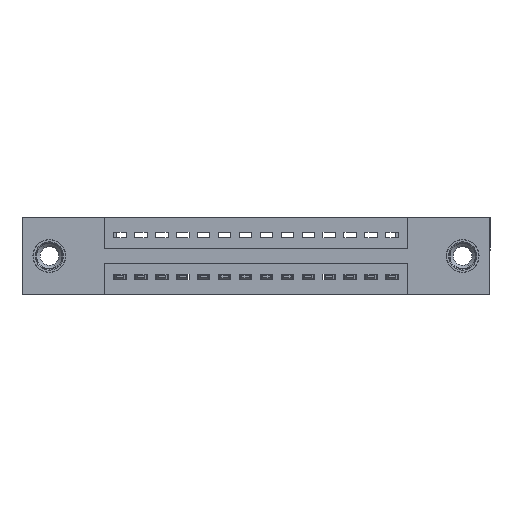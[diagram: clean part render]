
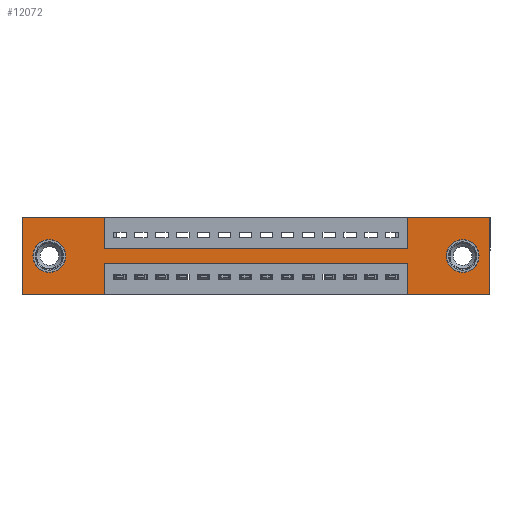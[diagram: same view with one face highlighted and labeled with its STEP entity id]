
A CAD part, front view. The second image highlights one B-rep face of the part: STEP entity #12072.
In plain terms, the highlighted planar face has unit normal (0, -1, 0).
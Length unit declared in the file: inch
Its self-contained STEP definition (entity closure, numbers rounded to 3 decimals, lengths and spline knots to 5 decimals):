
#70 = DIRECTION ( 'NONE',  ( 0., 1., 0. ) ) ;
#460 = AXIS2_PLACEMENT_3D ( 'NONE', #9441, #3684, #16946 ) ;
#713 = ORIENTED_EDGE ( 'NONE', *, *, #5972, .T. ) ;
#803 = ORIENTED_EDGE ( 'NONE', *, *, #4279, .F. ) ;
#848 = VERTEX_POINT ( 'NONE', #864 ) ;
#864 = CARTESIAN_POINT ( 'NONE',  ( 0., 0., 0. ) ) ;
#1004 = CARTESIAN_POINT ( 'NONE',  ( 0.3925, 0., -0.15 ) ) ;
#1243 = CARTESIAN_POINT ( 'NONE',  ( 2.235, 0., -0.37 ) ) ;
#1467 = ORIENTED_EDGE ( 'NONE', *, *, #2951, .F. ) ;
#1725 = VERTEX_POINT ( 'NONE', #14368 ) ;
#1738 = ORIENTED_EDGE ( 'NONE', *, *, #15918, .F. ) ;
#1948 = VERTEX_POINT ( 'NONE', #15063 ) ;
#2134 = CIRCLE ( 'NONE', #8075, 0.078 ) ;
#2428 = AXIS2_PLACEMENT_3D ( 'NONE', #12724, #17156, #8420 ) ;
#2469 = DIRECTION ( 'NONE',  ( 0., 0., 1. ) ) ;
#2610 = VECTOR ( 'NONE', #10086, 39.37008 ) ;
#2672 = CARTESIAN_POINT ( 'NONE',  ( 0.3925, 0., 0. ) ) ;
#2743 = VERTEX_POINT ( 'NONE', #13934 ) ;
#2900 = DIRECTION ( 'NONE',  ( 0., 0., 1. ) ) ;
#2901 = CARTESIAN_POINT ( 'NONE',  ( 1.8425, 0., -0.15 ) ) ;
#2913 = VECTOR ( 'NONE', #6463, 39.37008 ) ;
#2951 = EDGE_CURVE ( 'NONE', #15382, #3412, #18261, .T. ) ;
#3011 = CARTESIAN_POINT ( 'NONE',  ( 2.105, 0., -0.107 ) ) ;
#3070 = CARTESIAN_POINT ( 'NONE',  ( 1.8425, 0., -0.37 ) ) ;
#3412 = VERTEX_POINT ( 'NONE', #1243 ) ;
#3511 = DIRECTION ( 'NONE',  ( 0., 0., 1. ) ) ;
#3582 = EDGE_LOOP ( 'NONE', ( #16602, #17034 ) ) ;
#3594 = LINE ( 'NONE', #12085, #9097 ) ;
#3684 = DIRECTION ( 'NONE',  ( 0., -1., 0. ) ) ;
#3958 = DIRECTION ( 'NONE',  ( 0., 1., 0. ) ) ;
#4279 = EDGE_CURVE ( 'NONE', #848, #5965, #17296, .T. ) ;
#4366 = AXIS2_PLACEMENT_3D ( 'NONE', #18136, #3958, #3511 ) ;
#4417 = VECTOR ( 'NONE', #6159, 39.37008 ) ;
#4729 = VERTEX_POINT ( 'NONE', #15032 ) ;
#4902 = EDGE_CURVE ( 'NONE', #5724, #7267, #16792, .T. ) ;
#4928 = CARTESIAN_POINT ( 'NONE',  ( 0., 0., 0. ) ) ;
#5136 = VERTEX_POINT ( 'NONE', #2901 ) ;
#5249 = VERTEX_POINT ( 'NONE', #10340 ) ;
#5515 = CARTESIAN_POINT ( 'NONE',  ( 0.3925, 0., -0.22 ) ) ;
#5569 = DIRECTION ( 'NONE',  ( 0., 0., -1. ) ) ;
#5599 = VECTOR ( 'NONE', #14789, 39.37008 ) ;
#5714 = CARTESIAN_POINT ( 'NONE',  ( 0.3925, 0., 0. ) ) ;
#5724 = VERTEX_POINT ( 'NONE', #3070 ) ;
#5726 = CARTESIAN_POINT ( 'NONE',  ( 0.3925, 0., -0.15 ) ) ;
#5784 = FACE_BOUND ( 'NONE', #3582, .T. ) ;
#5814 = VECTOR ( 'NONE', #12591, 39.37008 ) ;
#5965 = VERTEX_POINT ( 'NONE', #2672 ) ;
#5972 = EDGE_CURVE ( 'NONE', #16766, #5249, #2134, .T. ) ;
#6159 = DIRECTION ( 'NONE',  ( -1., 0., 0. ) ) ;
#6307 = LINE ( 'NONE', #17658, #9524 ) ;
#6326 = CIRCLE ( 'NONE', #2428, 0.078 ) ;
#6414 = EDGE_CURVE ( 'NONE', #3412, #5724, #12609, .T. ) ;
#6463 = DIRECTION ( 'NONE',  ( -1., 0., 0. ) ) ;
#6726 = PLANE ( 'NONE',  #460 ) ;
#7267 = VERTEX_POINT ( 'NONE', #7624 ) ;
#7563 = VECTOR ( 'NONE', #2469, 39.37008 ) ;
#7624 = CARTESIAN_POINT ( 'NONE',  ( 1.8425, 0., -0.22 ) ) ;
#7673 = DIRECTION ( 'NONE',  ( -1., 0., 0. ) ) ;
#8075 = AXIS2_PLACEMENT_3D ( 'NONE', #12919, #17288, #15666 ) ;
#8339 = LINE ( 'NONE', #1004, #5814 ) ;
#8417 = VERTEX_POINT ( 'NONE', #14760 ) ;
#8420 = DIRECTION ( 'NONE',  ( 0., 0., -1. ) ) ;
#8852 = EDGE_LOOP ( 'NONE', ( #18480, #1738, #18056, #14288, #1467, #11668, #10074, #9271, #14047, #803, #10194, #9444 ) ) ;
#9030 = FACE_OUTER_BOUND ( 'NONE', #8852, .T. ) ;
#9097 = VECTOR ( 'NONE', #9306, 39.37008 ) ;
#9103 = CARTESIAN_POINT ( 'NONE',  ( 0., 0., -0.37 ) ) ;
#9271 = ORIENTED_EDGE ( 'NONE', *, *, #17104, .F. ) ;
#9306 = DIRECTION ( 'NONE',  ( 1., 0., 0. ) ) ;
#9441 = CARTESIAN_POINT ( 'NONE',  ( 0., 0., -0.37 ) ) ;
#9444 = ORIENTED_EDGE ( 'NONE', *, *, #11579, .F. ) ;
#9524 = VECTOR ( 'NONE', #10372, 39.37008 ) ;
#10074 = ORIENTED_EDGE ( 'NONE', *, *, #16237, .F. ) ;
#10086 = DIRECTION ( 'NONE',  ( 0., 0., -1. ) ) ;
#10194 = ORIENTED_EDGE ( 'NONE', *, *, #13725, .F. ) ;
#10303 = CARTESIAN_POINT ( 'NONE',  ( 0.13, 0., -0.185 ) ) ;
#10338 = CARTESIAN_POINT ( 'NONE',  ( 0., 0., -0.37 ) ) ;
#10340 = CARTESIAN_POINT ( 'NONE',  ( 2.105, 0., -0.263 ) ) ;
#10372 = DIRECTION ( 'NONE',  ( 0., 0., 1. ) ) ;
#10735 = DIRECTION ( 'NONE',  ( 1., 0., 0. ) ) ;
#10777 = LINE ( 'NONE', #12716, #7563 ) ;
#10839 = LINE ( 'NONE', #5714, #2610 ) ;
#11579 = EDGE_CURVE ( 'NONE', #2743, #8417, #17233, .T. ) ;
#11668 = ORIENTED_EDGE ( 'NONE', *, *, #15838, .F. ) ;
#11759 = LINE ( 'NONE', #16451, #5599 ) ;
#12072 = ADVANCED_FACE ( 'NONE', ( #17714, #5784, #9030 ), #6726, .T. ) ;
#12085 = CARTESIAN_POINT ( 'NONE',  ( 0., 0., 0. ) ) ;
#12181 = VERTEX_POINT ( 'NONE', #5515 ) ;
#12414 = CARTESIAN_POINT ( 'NONE',  ( 2.235, 0., 0. ) ) ;
#12591 = DIRECTION ( 'NONE',  ( 1., 0., 0. ) ) ;
#12609 = LINE ( 'NONE', #10338, #4417 ) ;
#12669 = CARTESIAN_POINT ( 'NONE',  ( 1.8425, 0., -0.37 ) ) ;
#12716 = CARTESIAN_POINT ( 'NONE',  ( 0., 0., 0. ) ) ;
#12724 = CARTESIAN_POINT ( 'NONE',  ( 2.105, 0., -0.185 ) ) ;
#12798 = DIRECTION ( 'NONE',  ( 0., 0., 1. ) ) ;
#12891 = EDGE_CURVE ( 'NONE', #1725, #4729, #15106, .T. ) ;
#12919 = CARTESIAN_POINT ( 'NONE',  ( 2.105, 0., -0.185 ) ) ;
#13156 = EDGE_CURVE ( 'NONE', #4729, #1725, #16947, .T. ) ;
#13224 = VECTOR ( 'NONE', #5569, 39.37008 ) ;
#13247 = VERTEX_POINT ( 'NONE', #5726 ) ;
#13512 = CARTESIAN_POINT ( 'NONE',  ( 2.235, 0., 0. ) ) ;
#13618 = ORIENTED_EDGE ( 'NONE', *, *, #15512, .T. ) ;
#13725 = EDGE_CURVE ( 'NONE', #8417, #848, #10777, .T. ) ;
#13934 = CARTESIAN_POINT ( 'NONE',  ( 0.3925, 0., -0.37 ) ) ;
#14047 = ORIENTED_EDGE ( 'NONE', *, *, #18270, .F. ) ;
#14288 = ORIENTED_EDGE ( 'NONE', *, *, #6414, .F. ) ;
#14368 = CARTESIAN_POINT ( 'NONE',  ( 0.13, 0., -0.263 ) ) ;
#14760 = CARTESIAN_POINT ( 'NONE',  ( 0., 0., -0.37 ) ) ;
#14789 = DIRECTION ( 'NONE',  ( 0., 0., -1. ) ) ;
#15032 = CARTESIAN_POINT ( 'NONE',  ( 0.13, 0., -0.107 ) ) ;
#15063 = CARTESIAN_POINT ( 'NONE',  ( 1.8425, 0., 0. ) ) ;
#15106 = CIRCLE ( 'NONE', #16457, 0.078 ) ;
#15190 = CARTESIAN_POINT ( 'NONE',  ( 0.3925, 0., -0.22 ) ) ;
#15217 = EDGE_LOOP ( 'NONE', ( #713, #13618 ) ) ;
#15382 = VERTEX_POINT ( 'NONE', #12414 ) ;
#15434 = LINE ( 'NONE', #15190, #2913 ) ;
#15512 = EDGE_CURVE ( 'NONE', #5249, #16766, #6326, .T. ) ;
#15666 = DIRECTION ( 'NONE',  ( 0., 0., -1. ) ) ;
#15838 = EDGE_CURVE ( 'NONE', #1948, #15382, #3594, .T. ) ;
#15918 = EDGE_CURVE ( 'NONE', #7267, #12181, #15434, .T. ) ;
#16237 = EDGE_CURVE ( 'NONE', #5136, #1948, #6307, .T. ) ;
#16451 = CARTESIAN_POINT ( 'NONE',  ( 0.3925, 0., -0.37 ) ) ;
#16457 = AXIS2_PLACEMENT_3D ( 'NONE', #10303, #70, #2900 ) ;
#16602 = ORIENTED_EDGE ( 'NONE', *, *, #13156, .T. ) ;
#16766 = VERTEX_POINT ( 'NONE', #3011 ) ;
#16792 = LINE ( 'NONE', #12669, #18385 ) ;
#16946 = DIRECTION ( 'NONE',  ( 0., 0., -1. ) ) ;
#16947 = CIRCLE ( 'NONE', #4366, 0.078 ) ;
#17034 = ORIENTED_EDGE ( 'NONE', *, *, #12891, .T. ) ;
#17104 = EDGE_CURVE ( 'NONE', #13247, #5136, #8339, .T. ) ;
#17156 = DIRECTION ( 'NONE',  ( 0., 1., 0. ) ) ;
#17233 = LINE ( 'NONE', #9103, #17255 ) ;
#17255 = VECTOR ( 'NONE', #7673, 39.37008 ) ;
#17288 = DIRECTION ( 'NONE',  ( 0., 1., 0. ) ) ;
#17296 = LINE ( 'NONE', #4928, #17772 ) ;
#17658 = CARTESIAN_POINT ( 'NONE',  ( 1.8425, 0., 0. ) ) ;
#17714 = FACE_BOUND ( 'NONE', #15217, .T. ) ;
#17772 = VECTOR ( 'NONE', #10735, 39.37008 ) ;
#17855 = EDGE_CURVE ( 'NONE', #12181, #2743, #11759, .T. ) ;
#18056 = ORIENTED_EDGE ( 'NONE', *, *, #4902, .F. ) ;
#18136 = CARTESIAN_POINT ( 'NONE',  ( 0.13, 0., -0.185 ) ) ;
#18261 = LINE ( 'NONE', #13512, #13224 ) ;
#18270 = EDGE_CURVE ( 'NONE', #5965, #13247, #10839, .T. ) ;
#18385 = VECTOR ( 'NONE', #12798, 39.37008 ) ;
#18480 = ORIENTED_EDGE ( 'NONE', *, *, #17855, .F. ) ;
